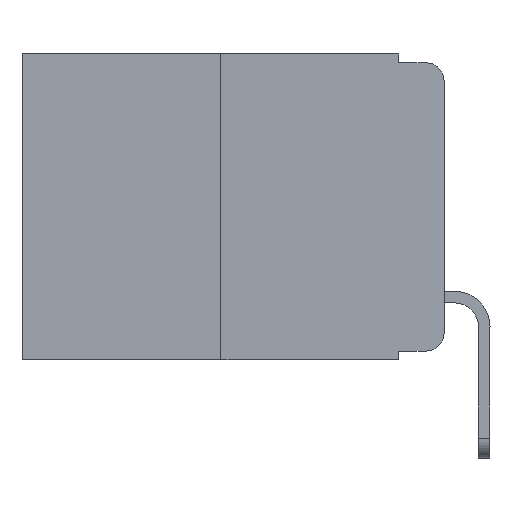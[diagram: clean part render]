
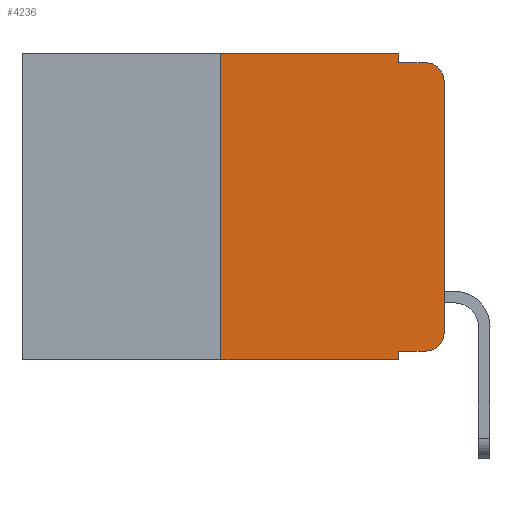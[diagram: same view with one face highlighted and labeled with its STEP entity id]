
A CAD part, left-side view. The second image highlights one B-rep face of the part: STEP entity #4236.
In plain terms, the highlighted planar face has unit normal (-1, 0, 0).
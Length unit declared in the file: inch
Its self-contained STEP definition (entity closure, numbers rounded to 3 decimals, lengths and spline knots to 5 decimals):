
#365 = CARTESIAN_POINT ( 'NONE',  ( 0., 0.25, 0. ) ) ;
#468 = ORIENTED_EDGE ( 'NONE', *, *, #14107, .F. ) ;
#1198 = CARTESIAN_POINT ( 'NONE',  ( 0., 0.051, -0.333 ) ) ;
#1271 = EDGE_CURVE ( 'NONE', #3812, #23439, #10716, .T. ) ;
#1777 = VECTOR ( 'NONE', #24819, 39.37008 ) ;
#2210 = LINE ( 'NONE', #6371, #16789 ) ;
#2284 = VERTEX_POINT ( 'NONE', #4852 ) ;
#2396 = LINE ( 'NONE', #1198, #1777 ) ;
#2720 = PLANE ( 'NONE',  #5598 ) ;
#2929 = CARTESIAN_POINT ( 'NONE',  ( 0., 0.02, -0.313 ) ) ;
#3177 = AXIS2_PLACEMENT_3D ( 'NONE', #22469, #10704, #24415 ) ;
#3575 = ORIENTED_EDGE ( 'NONE', *, *, #18326, .T. ) ;
#3812 = VERTEX_POINT ( 'NONE', #16957 ) ;
#4236 = ADVANCED_FACE ( 'NONE', ( #16068 ), #2720, .F. ) ;
#4287 = CIRCLE ( 'NONE', #19651, 0.02 ) ;
#4419 = ORIENTED_EDGE ( 'NONE', *, *, #18412, .T. ) ;
#4654 = CIRCLE ( 'NONE', #3177, 0.02 ) ;
#4707 = VERTEX_POINT ( 'NONE', #12291 ) ;
#4852 = CARTESIAN_POINT ( 'NONE',  ( 0., 0., -0.03 ) ) ;
#4932 = DIRECTION ( 'NONE',  ( 0., 0., -1. ) ) ;
#5054 = ORIENTED_EDGE ( 'NONE', *, *, #23790, .T. ) ;
#5598 = AXIS2_PLACEMENT_3D ( 'NONE', #20549, #8757, #22511 ) ;
#5682 = CARTESIAN_POINT ( 'NONE',  ( 0., 0.02, -0.01 ) ) ;
#6371 = CARTESIAN_POINT ( 'NONE',  ( 0., 0., 0. ) ) ;
#6761 = CARTESIAN_POINT ( 'NONE',  ( 0., 0.473, -0.343 ) ) ;
#7153 = CARTESIAN_POINT ( 'NONE',  ( 0., 0.051, -0.01 ) ) ;
#7994 = CARTESIAN_POINT ( 'NONE',  ( 0., 0., -0.313 ) ) ;
#8400 = DIRECTION ( 'NONE',  ( 0., 0., 1. ) ) ;
#8757 = DIRECTION ( 'NONE',  ( 1., 0., 0. ) ) ;
#8824 = VECTOR ( 'NONE', #22526, 39.37008 ) ;
#9507 = EDGE_CURVE ( 'NONE', #10942, #24615, #9868, .T. ) ;
#9868 = LINE ( 'NONE', #20512, #24894 ) ;
#9955 = ORIENTED_EDGE ( 'NONE', *, *, #21374, .T. ) ;
#10197 = EDGE_CURVE ( 'NONE', #12083, #15031, #20026, .T. ) ;
#10339 = ORIENTED_EDGE ( 'NONE', *, *, #10197, .F. ) ;
#10655 = DIRECTION ( 'NONE',  ( 0., 0., -1. ) ) ;
#10704 = DIRECTION ( 'NONE',  ( -1., 0., 0. ) ) ;
#10716 = LINE ( 'NONE', #12438, #20565 ) ;
#10942 = VERTEX_POINT ( 'NONE', #7153 ) ;
#11917 = ORIENTED_EDGE ( 'NONE', *, *, #21880, .T. ) ;
#12083 = VERTEX_POINT ( 'NONE', #20802 ) ;
#12088 = VECTOR ( 'NONE', #14577, 39.37008 ) ;
#12291 = CARTESIAN_POINT ( 'NONE',  ( 0., 0.02, -0.333 ) ) ;
#12430 = DIRECTION ( 'NONE',  ( 0., -1., 0. ) ) ;
#12438 = CARTESIAN_POINT ( 'NONE',  ( 0., 0.473, 0. ) ) ;
#12589 = CARTESIAN_POINT ( 'NONE',  ( 0., 0.051, 0. ) ) ;
#13422 = VERTEX_POINT ( 'NONE', #7994 ) ;
#13612 = CARTESIAN_POINT ( 'NONE',  ( 0., 0.051, 0. ) ) ;
#14073 = LINE ( 'NONE', #6761, #8824 ) ;
#14107 = EDGE_CURVE ( 'NONE', #22912, #3812, #20149, .T. ) ;
#14577 = DIRECTION ( 'NONE',  ( 0., 0., -1. ) ) ;
#14948 = VECTOR ( 'NONE', #20182, 39.37008 ) ;
#15031 = VERTEX_POINT ( 'NONE', #21083 ) ;
#15447 = VECTOR ( 'NONE', #10655, 39.37008 ) ;
#16068 = FACE_OUTER_BOUND ( 'NONE', #22310, .T. ) ;
#16508 = CARTESIAN_POINT ( 'NONE',  ( 0., 0.051, 0. ) ) ;
#16789 = VECTOR ( 'NONE', #8400, 39.37008 ) ;
#16790 = DIRECTION ( 'NONE',  ( -1., 0., 0. ) ) ;
#16849 = ORIENTED_EDGE ( 'NONE', *, *, #1271, .F. ) ;
#16957 = CARTESIAN_POINT ( 'NONE',  ( 0., 0.25, 0. ) ) ;
#18233 = EDGE_CURVE ( 'NONE', #23439, #10942, #23124, .T. ) ;
#18326 = EDGE_CURVE ( 'NONE', #4707, #13422, #4287, .T. ) ;
#18412 = EDGE_CURVE ( 'NONE', #12083, #4707, #2396, .T. ) ;
#19651 = AXIS2_PLACEMENT_3D ( 'NONE', #2929, #16790, #4932 ) ;
#20026 = LINE ( 'NONE', #16508, #15447 ) ;
#20149 = LINE ( 'NONE', #365, #14948 ) ;
#20182 = DIRECTION ( 'NONE',  ( 0., 0., 1. ) ) ;
#20512 = CARTESIAN_POINT ( 'NONE',  ( 0., 0.051, -0.01 ) ) ;
#20549 = CARTESIAN_POINT ( 'NONE',  ( 0., 0.473, 0. ) ) ;
#20565 = VECTOR ( 'NONE', #12430, 39.37008 ) ;
#20802 = CARTESIAN_POINT ( 'NONE',  ( 0., 0.051, -0.333 ) ) ;
#20947 = ORIENTED_EDGE ( 'NONE', *, *, #18233, .F. ) ;
#21083 = CARTESIAN_POINT ( 'NONE',  ( 0., 0.051, -0.343 ) ) ;
#21351 = CARTESIAN_POINT ( 'NONE',  ( 0., 0.25, -0.343 ) ) ;
#21374 = EDGE_CURVE ( 'NONE', #22912, #15031, #14073, .T. ) ;
#21880 = EDGE_CURVE ( 'NONE', #13422, #2284, #2210, .T. ) ;
#22310 = EDGE_LOOP ( 'NONE', ( #11917, #5054, #25020, #20947, #16849, #468, #9955, #10339, #4419, #3575 ) ) ;
#22469 = CARTESIAN_POINT ( 'NONE',  ( 0., 0.02, -0.03 ) ) ;
#22473 = DIRECTION ( 'NONE',  ( 0., -1., 0. ) ) ;
#22511 = DIRECTION ( 'NONE',  ( 0., 0., -1. ) ) ;
#22526 = DIRECTION ( 'NONE',  ( 0., -1., 0. ) ) ;
#22912 = VERTEX_POINT ( 'NONE', #21351 ) ;
#23124 = LINE ( 'NONE', #12589, #12088 ) ;
#23439 = VERTEX_POINT ( 'NONE', #13612 ) ;
#23790 = EDGE_CURVE ( 'NONE', #2284, #24615, #4654, .T. ) ;
#24415 = DIRECTION ( 'NONE',  ( 0., 0., -1. ) ) ;
#24615 = VERTEX_POINT ( 'NONE', #5682 ) ;
#24819 = DIRECTION ( 'NONE',  ( 0., -1., 0. ) ) ;
#24894 = VECTOR ( 'NONE', #22473, 39.37008 ) ;
#25020 = ORIENTED_EDGE ( 'NONE', *, *, #9507, .F. ) ;
